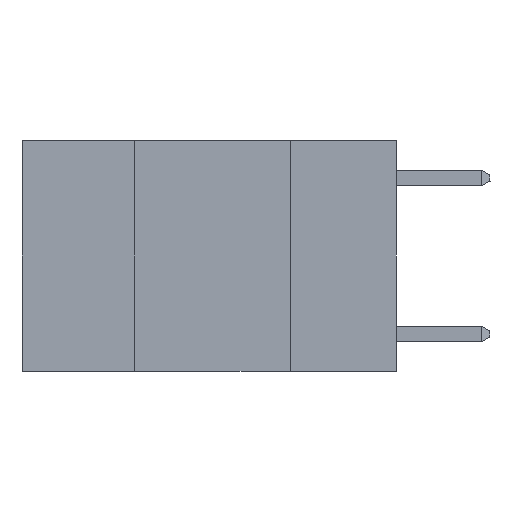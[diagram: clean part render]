
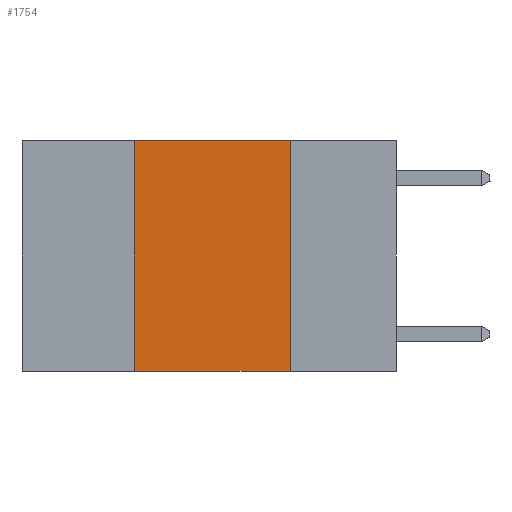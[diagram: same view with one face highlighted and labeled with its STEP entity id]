
A CAD part, left-side view. The second image highlights one B-rep face of the part: STEP entity #1754.
In plain terms, the highlighted planar face has unit normal (-1, 0, 0).
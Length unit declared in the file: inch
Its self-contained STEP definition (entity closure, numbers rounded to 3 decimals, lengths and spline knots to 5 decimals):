
#96 = CARTESIAN_POINT ( 'NONE',  ( 0., 0.17, 0. ) ) ;
#173 = ORIENTED_EDGE ( 'NONE', *, *, #1490, .T. ) ;
#706 = AXIS2_PLACEMENT_3D ( 'NONE', #2920, #9201, #3825 ) ;
#981 = VECTOR ( 'NONE', #1733, 39.37008 ) ;
#1490 = EDGE_CURVE ( 'NONE', #5172, #8391, #2473, .T. ) ;
#1617 = DIRECTION ( 'NONE',  ( 0., -1., 0. ) ) ;
#1733 = DIRECTION ( 'NONE',  ( 0., -1., 0. ) ) ;
#1754 = ADVANCED_FACE ( 'NONE', ( #8931 ), #8273, .F. ) ;
#2473 = LINE ( 'NONE', #7878, #2762 ) ;
#2762 = VECTOR ( 'NONE', #1617, 39.37008 ) ;
#2920 = CARTESIAN_POINT ( 'NONE',  ( 0., 0.6, 0. ) ) ;
#3110 = CARTESIAN_POINT ( 'NONE',  ( 0., 0.17, -0.37 ) ) ;
#3282 = CARTESIAN_POINT ( 'NONE',  ( 0., 0.17, 0. ) ) ;
#3825 = DIRECTION ( 'NONE',  ( 0., 0., -1. ) ) ;
#5026 = EDGE_CURVE ( 'NONE', #8188, #8391, #7707, .T. ) ;
#5172 = VERTEX_POINT ( 'NONE', #11617 ) ;
#5174 = EDGE_CURVE ( 'NONE', #6758, #8188, #5755, .T. ) ;
#5245 = CARTESIAN_POINT ( 'NONE',  ( 0., 0.42, 0. ) ) ;
#5343 = VECTOR ( 'NONE', #5964, 39.37008 ) ;
#5567 = EDGE_LOOP ( 'NONE', ( #5918, #6482, #8307, #173 ) ) ;
#5755 = LINE ( 'NONE', #10694, #981 ) ;
#5918 = ORIENTED_EDGE ( 'NONE', *, *, #5026, .F. ) ;
#5964 = DIRECTION ( 'NONE',  ( 0., 0., -1. ) ) ;
#6482 = ORIENTED_EDGE ( 'NONE', *, *, #5174, .F. ) ;
#6758 = VERTEX_POINT ( 'NONE', #11348 ) ;
#7707 = LINE ( 'NONE', #3282, #5343 ) ;
#7878 = CARTESIAN_POINT ( 'NONE',  ( 0., 0.6, -0.37 ) ) ;
#8115 = VECTOR ( 'NONE', #9759, 39.37008 ) ;
#8188 = VERTEX_POINT ( 'NONE', #96 ) ;
#8273 = PLANE ( 'NONE',  #706 ) ;
#8307 = ORIENTED_EDGE ( 'NONE', *, *, #9403, .F. ) ;
#8391 = VERTEX_POINT ( 'NONE', #3110 ) ;
#8931 = FACE_OUTER_BOUND ( 'NONE', #5567, .T. ) ;
#9201 = DIRECTION ( 'NONE',  ( 1., 0., 0. ) ) ;
#9403 = EDGE_CURVE ( 'NONE', #5172, #6758, #10527, .T. ) ;
#9759 = DIRECTION ( 'NONE',  ( 0., 0., 1. ) ) ;
#10527 = LINE ( 'NONE', #5245, #8115 ) ;
#10694 = CARTESIAN_POINT ( 'NONE',  ( 0., 0.6, 0. ) ) ;
#11348 = CARTESIAN_POINT ( 'NONE',  ( 0., 0.42, 0. ) ) ;
#11617 = CARTESIAN_POINT ( 'NONE',  ( 0., 0.42, -0.37 ) ) ;
